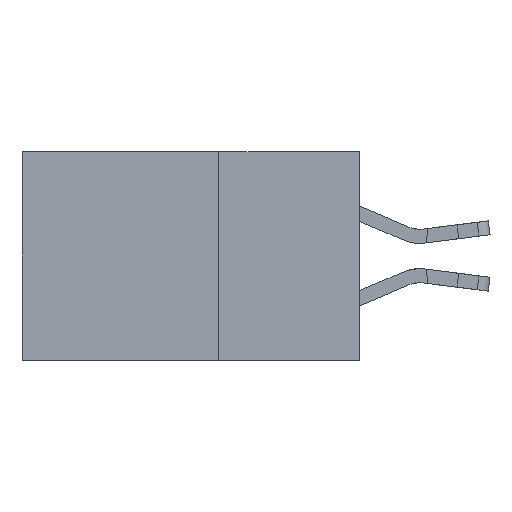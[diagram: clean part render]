
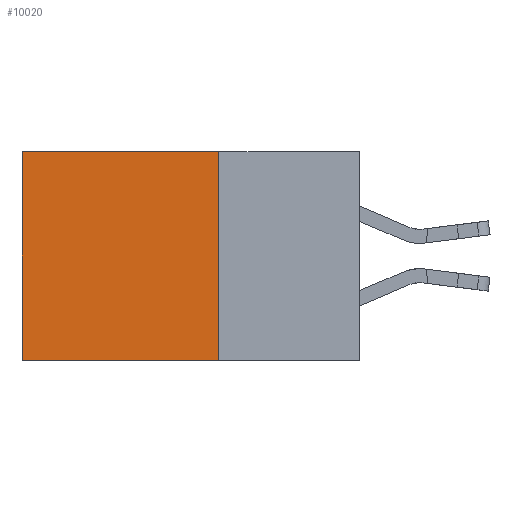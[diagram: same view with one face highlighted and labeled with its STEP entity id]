
A CAD part, left-side view. The second image highlights one B-rep face of the part: STEP entity #10020.
In plain terms, the highlighted planar face has unit normal (-1, 0, 0).
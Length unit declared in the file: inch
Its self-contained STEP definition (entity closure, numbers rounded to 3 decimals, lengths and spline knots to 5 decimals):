
#170 = DIRECTION ( 'NONE',  ( 0., 0., -1. ) ) ;
#671 = FACE_OUTER_BOUND ( 'NONE', #19613, .T. ) ;
#1677 = VECTOR ( 'NONE', #11490, 39.37008 ) ;
#2913 = CARTESIAN_POINT ( 'NONE',  ( 0.2875, 0.25, -0.37 ) ) ;
#3172 = AXIS2_PLACEMENT_3D ( 'NONE', #11889, #8951, #28814 ) ;
#3265 = ORIENTED_EDGE ( 'NONE', *, *, #10480, .F. ) ;
#5148 = VERTEX_POINT ( 'NONE', #2913 ) ;
#5360 = DIRECTION ( 'NONE',  ( 0., 1., 0. ) ) ;
#5652 = PLANE ( 'NONE',  #3172 ) ;
#7089 = CARTESIAN_POINT ( 'NONE',  ( 0.2875, 0.25, -0.37 ) ) ;
#8951 = DIRECTION ( 'NONE',  ( 1., 0., 0. ) ) ;
#9505 = EDGE_CURVE ( 'NONE', #11080, #29899, #11393, .T. ) ;
#10020 = ADVANCED_FACE ( 'NONE', ( #671 ), #5652, .F. ) ;
#10480 = EDGE_CURVE ( 'NONE', #25148, #5148, #25659, .T. ) ;
#11080 = VERTEX_POINT ( 'NONE', #22626 ) ;
#11248 = CARTESIAN_POINT ( 'NONE',  ( 0.2875, 0.25, 0. ) ) ;
#11393 = LINE ( 'NONE', #31425, #29554 ) ;
#11490 = DIRECTION ( 'NONE',  ( 0., 0., -1. ) ) ;
#11889 = CARTESIAN_POINT ( 'NONE',  ( 0.2875, 0.25, 0. ) ) ;
#14192 = LINE ( 'NONE', #11248, #22178 ) ;
#15220 = DIRECTION ( 'NONE',  ( 0., 1., 0. ) ) ;
#18735 = EDGE_CURVE ( 'NONE', #5148, #29899, #21100, .T. ) ;
#19613 = EDGE_LOOP ( 'NONE', ( #34506, #28609, #3265, #25142 ) ) ;
#21100 = LINE ( 'NONE', #7089, #24790 ) ;
#22178 = VECTOR ( 'NONE', #5360, 39.37008 ) ;
#22626 = CARTESIAN_POINT ( 'NONE',  ( 0.2875, 0.6, 0. ) ) ;
#24790 = VECTOR ( 'NONE', #15220, 39.37008 ) ;
#25142 = ORIENTED_EDGE ( 'NONE', *, *, #31743, .T. ) ;
#25148 = VERTEX_POINT ( 'NONE', #28579 ) ;
#25659 = LINE ( 'NONE', #28591, #1677 ) ;
#28579 = CARTESIAN_POINT ( 'NONE',  ( 0.2875, 0.25, 0. ) ) ;
#28591 = CARTESIAN_POINT ( 'NONE',  ( 0.2875, 0.25, 0. ) ) ;
#28609 = ORIENTED_EDGE ( 'NONE', *, *, #18735, .F. ) ;
#28814 = DIRECTION ( 'NONE',  ( 0., 0., -1. ) ) ;
#29554 = VECTOR ( 'NONE', #170, 39.37008 ) ;
#29866 = CARTESIAN_POINT ( 'NONE',  ( 0.2875, 0.6, -0.37 ) ) ;
#29899 = VERTEX_POINT ( 'NONE', #29866 ) ;
#31425 = CARTESIAN_POINT ( 'NONE',  ( 0.2875, 0.6, 0. ) ) ;
#31743 = EDGE_CURVE ( 'NONE', #25148, #11080, #14192, .T. ) ;
#34506 = ORIENTED_EDGE ( 'NONE', *, *, #9505, .T. ) ;
